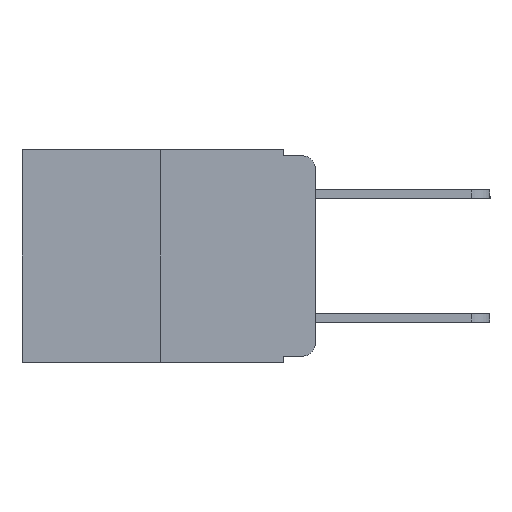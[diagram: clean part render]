
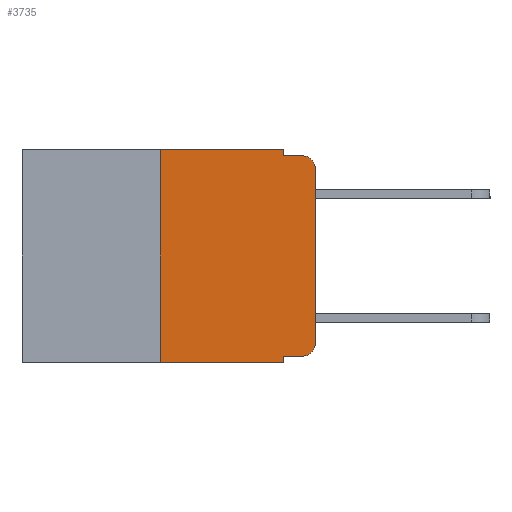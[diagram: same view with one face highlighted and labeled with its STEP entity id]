
A CAD part, left-side view. The second image highlights one B-rep face of the part: STEP entity #3735.
In plain terms, the highlighted planar face has unit normal (-1, 0, 0).
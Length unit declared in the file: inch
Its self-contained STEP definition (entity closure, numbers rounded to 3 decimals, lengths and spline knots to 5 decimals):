
#164 = CARTESIAN_POINT ( 'NONE',  ( 0., 0.25, 0. ) ) ;
#2093 = CARTESIAN_POINT ( 'NONE',  ( 0., 0., 0. ) ) ;
#2144 = AXIS2_PLACEMENT_3D ( 'NONE', #7286, #20416, #9182 ) ;
#3442 = CARTESIAN_POINT ( 'NONE',  ( 0., 0.25, 0. ) ) ;
#3735 = ADVANCED_FACE ( 'NONE', ( #22063 ), #21012, .F. ) ;
#4102 = CARTESIAN_POINT ( 'NONE',  ( 0., 0.051, 0. ) ) ;
#4199 = DIRECTION ( 'NONE',  ( 0., 0., 1. ) ) ;
#5432 = ORIENTED_EDGE ( 'NONE', *, *, #11390, .F. ) ;
#5561 = EDGE_CURVE ( 'NONE', #15515, #16893, #20766, .T. ) ;
#5669 = VECTOR ( 'NONE', #17432, 39.37008 ) ;
#5679 = DIRECTION ( 'NONE',  ( 0., -1., 0. ) ) ;
#6046 = ORIENTED_EDGE ( 'NONE', *, *, #18750, .T. ) ;
#6055 = DIRECTION ( 'NONE',  ( 0., 0., -1. ) ) ;
#6056 = CARTESIAN_POINT ( 'NONE',  ( 0., 0.051, 0. ) ) ;
#6116 = VERTEX_POINT ( 'NONE', #3442 ) ;
#6282 = LINE ( 'NONE', #2093, #5669 ) ;
#6529 = VERTEX_POINT ( 'NONE', #8530 ) ;
#6756 = CARTESIAN_POINT ( 'NONE',  ( 0., 0., -0.03 ) ) ;
#6929 = ORIENTED_EDGE ( 'NONE', *, *, #7456, .F. ) ;
#7226 = CARTESIAN_POINT ( 'NONE',  ( 0., 0.051, -0.01 ) ) ;
#7286 = CARTESIAN_POINT ( 'NONE',  ( 0., 0.02, -0.03 ) ) ;
#7456 = EDGE_CURVE ( 'NONE', #6116, #6529, #19516, .T. ) ;
#7642 = CARTESIAN_POINT ( 'NONE',  ( 0., 0.473, 0. ) ) ;
#8047 = VERTEX_POINT ( 'NONE', #11309 ) ;
#8105 = DIRECTION ( 'NONE',  ( 0., 0., -1. ) ) ;
#8530 = CARTESIAN_POINT ( 'NONE',  ( 0., 0.051, 0. ) ) ;
#8698 = ORIENTED_EDGE ( 'NONE', *, *, #21982, .F. ) ;
#8824 = LINE ( 'NONE', #164, #14493 ) ;
#9182 = DIRECTION ( 'NONE',  ( 0., 0., -1. ) ) ;
#9190 = DIRECTION ( 'NONE',  ( -1., 0., 0. ) ) ;
#9228 = VERTEX_POINT ( 'NONE', #13208 ) ;
#9552 = DIRECTION ( 'NONE',  ( 0., -1., 0. ) ) ;
#10269 = VECTOR ( 'NONE', #8105, 39.37008 ) ;
#11084 = EDGE_CURVE ( 'NONE', #21205, #16032, #15357, .T. ) ;
#11128 = LINE ( 'NONE', #16978, #14965 ) ;
#11309 = CARTESIAN_POINT ( 'NONE',  ( 0., 0.051, -0.343 ) ) ;
#11390 = EDGE_CURVE ( 'NONE', #9228, #6116, #8824, .T. ) ;
#11415 = ORIENTED_EDGE ( 'NONE', *, *, #14902, .T. ) ;
#11853 = VECTOR ( 'NONE', #14867, 39.37008 ) ;
#12005 = ORIENTED_EDGE ( 'NONE', *, *, #11084, .T. ) ;
#12317 = ORIENTED_EDGE ( 'NONE', *, *, #18234, .F. ) ;
#12395 = CARTESIAN_POINT ( 'NONE',  ( 0., 0., -0.313 ) ) ;
#12547 = EDGE_LOOP ( 'NONE', ( #11415, #12005, #8698, #21022, #6929, #5432, #6046, #12317, #22778, #15877 ) ) ;
#12912 = LINE ( 'NONE', #6056, #21628 ) ;
#13208 = CARTESIAN_POINT ( 'NONE',  ( 0., 0.25, -0.343 ) ) ;
#13639 = CARTESIAN_POINT ( 'NONE',  ( 0., 0.473, 0. ) ) ;
#13756 = CARTESIAN_POINT ( 'NONE',  ( 0., 0.02, -0.333 ) ) ;
#14493 = VECTOR ( 'NONE', #4199, 39.37008 ) ;
#14600 = VECTOR ( 'NONE', #9552, 39.37008 ) ;
#14867 = DIRECTION ( 'NONE',  ( 0., -1., 0. ) ) ;
#14902 = EDGE_CURVE ( 'NONE', #20015, #21205, #6282, .T. ) ;
#14965 = VECTOR ( 'NONE', #5679, 39.37008 ) ;
#15357 = CIRCLE ( 'NONE', #2144, 0.02 ) ;
#15515 = VERTEX_POINT ( 'NONE', #24584 ) ;
#15877 = ORIENTED_EDGE ( 'NONE', *, *, #22861, .T. ) ;
#15884 = VECTOR ( 'NONE', #20862, 39.37008 ) ;
#16032 = VERTEX_POINT ( 'NONE', #22455 ) ;
#16047 = AXIS2_PLACEMENT_3D ( 'NONE', #20425, #9190, #22278 ) ;
#16226 = AXIS2_PLACEMENT_3D ( 'NONE', #13639, #17396, #6055 ) ;
#16839 = LINE ( 'NONE', #7226, #11853 ) ;
#16893 = VERTEX_POINT ( 'NONE', #13756 ) ;
#16978 = CARTESIAN_POINT ( 'NONE',  ( 0., 0.473, -0.343 ) ) ;
#17396 = DIRECTION ( 'NONE',  ( 1., 0., 0. ) ) ;
#17432 = DIRECTION ( 'NONE',  ( 0., 0., 1. ) ) ;
#17650 = EDGE_CURVE ( 'NONE', #6529, #20322, #20215, .T. ) ;
#18234 = EDGE_CURVE ( 'NONE', #15515, #8047, #12912, .T. ) ;
#18728 = CARTESIAN_POINT ( 'NONE',  ( 0., 0.051, -0.01 ) ) ;
#18750 = EDGE_CURVE ( 'NONE', #9228, #8047, #11128, .T. ) ;
#19090 = CIRCLE ( 'NONE', #16047, 0.02 ) ;
#19516 = LINE ( 'NONE', #7642, #14600 ) ;
#20015 = VERTEX_POINT ( 'NONE', #12395 ) ;
#20215 = LINE ( 'NONE', #4102, #10269 ) ;
#20322 = VERTEX_POINT ( 'NONE', #18728 ) ;
#20416 = DIRECTION ( 'NONE',  ( -1., 0., 0. ) ) ;
#20425 = CARTESIAN_POINT ( 'NONE',  ( 0., 0.02, -0.313 ) ) ;
#20766 = LINE ( 'NONE', #22629, #15884 ) ;
#20862 = DIRECTION ( 'NONE',  ( 0., -1., 0. ) ) ;
#21012 = PLANE ( 'NONE',  #16226 ) ;
#21022 = ORIENTED_EDGE ( 'NONE', *, *, #17650, .F. ) ;
#21096 = DIRECTION ( 'NONE',  ( 0., 0., -1. ) ) ;
#21205 = VERTEX_POINT ( 'NONE', #6756 ) ;
#21628 = VECTOR ( 'NONE', #21096, 39.37008 ) ;
#21982 = EDGE_CURVE ( 'NONE', #20322, #16032, #16839, .T. ) ;
#22063 = FACE_OUTER_BOUND ( 'NONE', #12547, .T. ) ;
#22278 = DIRECTION ( 'NONE',  ( 0., 0., -1. ) ) ;
#22455 = CARTESIAN_POINT ( 'NONE',  ( 0., 0.02, -0.01 ) ) ;
#22629 = CARTESIAN_POINT ( 'NONE',  ( 0., 0.051, -0.333 ) ) ;
#22778 = ORIENTED_EDGE ( 'NONE', *, *, #5561, .T. ) ;
#22861 = EDGE_CURVE ( 'NONE', #16893, #20015, #19090, .T. ) ;
#24584 = CARTESIAN_POINT ( 'NONE',  ( 0., 0.051, -0.333 ) ) ;
